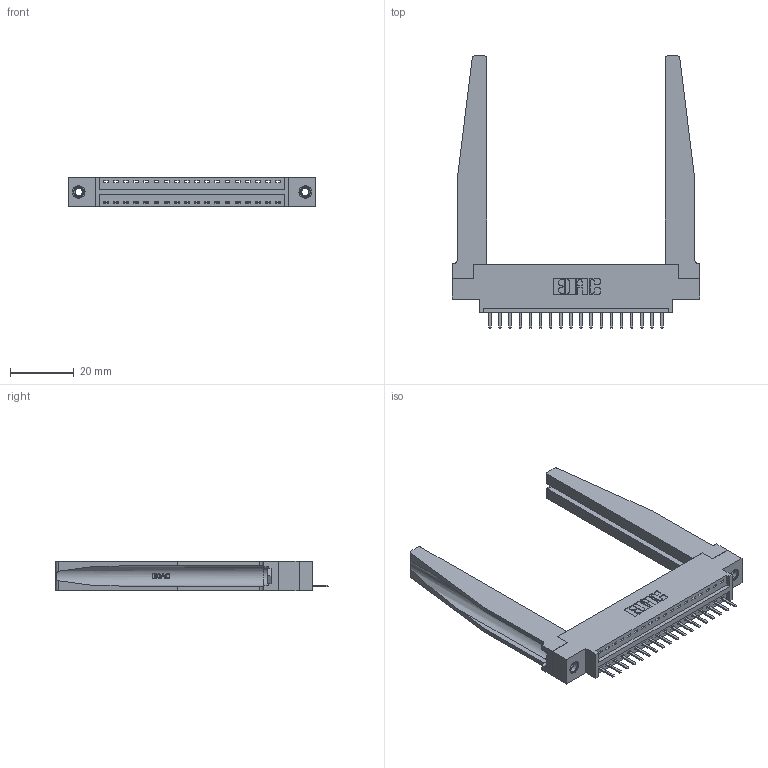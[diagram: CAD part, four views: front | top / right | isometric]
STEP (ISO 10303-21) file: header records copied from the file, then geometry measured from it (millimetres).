
FILE_DESCRIPTION (( 'STEP AP203' ), '1' );
FILE_NAME ('396-018-520-678.STEP', '2019-10-26T19:29:43', ( '' ), ( '' ), 'SwSTEP 2.0', 'SolidWorks 2016', '' );
FILE_SCHEMA (( 'CONFIG_CONTROL_DESIGN' ));
Length unit declared in the file: inch
Products named in the file (5): 345-250-001_345-250-001-102; 346-220-078_345-220-078; 346 Part_0.170 Offset - 0.156 Dia-TH; 345-292-001_345-293-120; 396-018-520-678
Assembly tree (23 placements, depth 2):
  396-018-520-678
    346 Part_0.170 Offset - 0.156 Dia-TH
    345-292-001_345-293-120  x18
    346-220-078_345-220-078  x2
    345-250-001_345-250-001-102  x2
Bounding box: 77.72 x 85.29 x 9.4 mm (x, y, z)
Volume: 13977 mm3; surface area: 15102.9 mm2
Topology: 23 solids, 23 shells, 1476 faces, 4261 edges, 2782 vertices
Faces by surface type: plane 978, cylinder 446, bspline 36, cone 12, torus 4
Entity records: 19396 total; most frequent: CARTESIAN_POINT 4257, ORIENTED_EDGE 3086, DIRECTION 2757, EDGE_CURVE 1543, LINE 1241, VECTOR 1241, VERTEX_POINT 1020, AXIS2_PLACEMENT_3D 758
